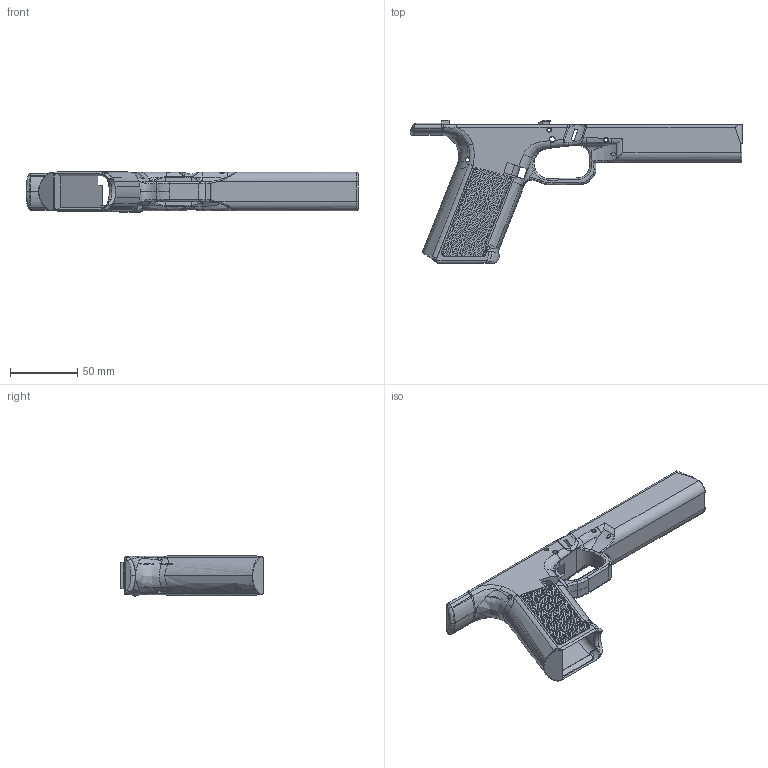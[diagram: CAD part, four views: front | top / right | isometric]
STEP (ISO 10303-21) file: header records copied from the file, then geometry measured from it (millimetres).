
FILE_DESCRIPTION(/* description */ (''),/* implementation_level */ '2;1');
FILE_NAME(/* name */ 'G17 Big Chungus Slick.step',/* time_stamp */ '2021-04-09T08:55:46-06:00',/* author */ (''),/* organization */ (''),/* preprocessor_version */ 'ST-DEVELOPER v18.1',/* originating_system */ 'Autodesk Translation Framework v9.10.0.1330',/* authorisation */ '');
FILE_SCHEMA (('AUTOMOTIVE_DESIGN { 1 0 10303 214 3 1 1 }'));
Products named in the file (1): G17 Big Chungus Slick
Bounding box: 247.28 x 106.5 x 30.34 mm (x, y, z)
Volume: 133516.5 mm3; surface area: 62494.6 mm2
Topology: 1 solids, 3 shells, 3250 faces, 8762 edges, 5703 vertices
Faces by surface type: plane 1645, bspline 1387, cylinder 153, torus 40, sphere 16, cone 9
Full cylindrical faces by diameter (mm): 2 x2, 3 x4, 3.2 x2, 4 x2, 9.55 x2
Entity records: 128371 total; most frequent: CARTESIAN_POINT 59476, ORIENTED_EDGE 17504, DIRECTION 10285, EDGE_CURVE 8752, VERTEX_POINT 5704, LINE 5347, VECTOR 5347, EDGE_LOOP 3480
